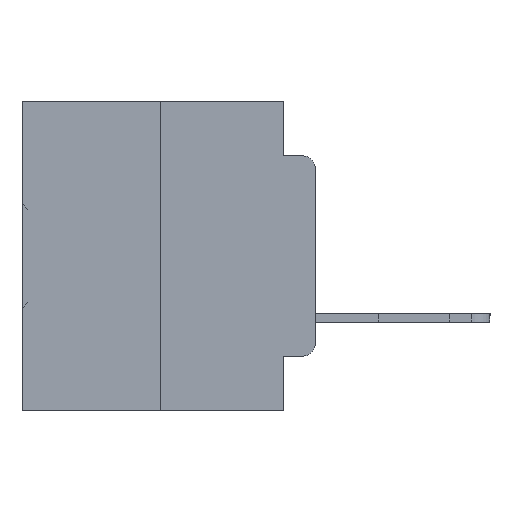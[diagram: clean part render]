
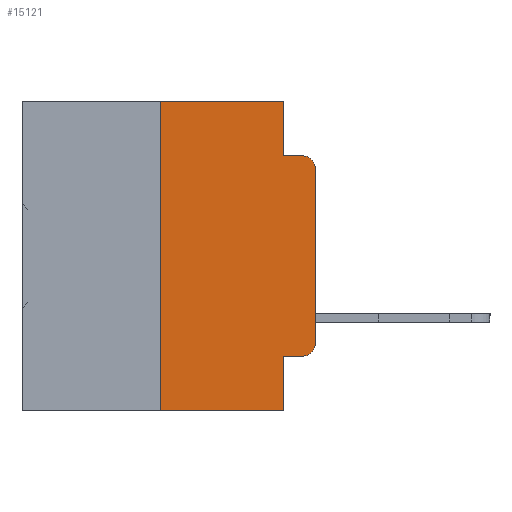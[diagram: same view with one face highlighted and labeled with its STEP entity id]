
A CAD part, left-side view. The second image highlights one B-rep face of the part: STEP entity #15121.
In plain terms, the highlighted planar face has unit normal (-1, 0, 0).
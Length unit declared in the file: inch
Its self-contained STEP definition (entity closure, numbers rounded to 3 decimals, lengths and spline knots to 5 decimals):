
#551 = DIRECTION ( 'NONE',  ( 0., 0., 1. ) ) ;
#1004 = VERTEX_POINT ( 'NONE', #1181 ) ;
#1014 = CARTESIAN_POINT ( 'NONE',  ( 0., 0.051, -0.5 ) ) ;
#1134 = ORIENTED_EDGE ( 'NONE', *, *, #14506, .F. ) ;
#1181 = CARTESIAN_POINT ( 'NONE',  ( 0., 0.051, 0. ) ) ;
#1571 = EDGE_CURVE ( 'NONE', #15474, #32613, #20621, .T. ) ;
#1595 = CARTESIAN_POINT ( 'NONE',  ( 0., 0.051, 0. ) ) ;
#1701 = LINE ( 'NONE', #3134, #15509 ) ;
#2560 = CARTESIAN_POINT ( 'NONE',  ( 0., 0., 0. ) ) ;
#3134 = CARTESIAN_POINT ( 'NONE',  ( 0., 0.051, 0. ) ) ;
#4135 = ORIENTED_EDGE ( 'NONE', *, *, #34524, .T. ) ;
#4772 = DIRECTION ( 'NONE',  ( -1., 0., 0. ) ) ;
#4811 = EDGE_CURVE ( 'NONE', #16087, #28136, #8216, .T. ) ;
#5241 = EDGE_CURVE ( 'NONE', #15474, #28136, #1701, .T. ) ;
#6023 = VECTOR ( 'NONE', #12230, 39.37008 ) ;
#6100 = VECTOR ( 'NONE', #30065, 39.37008 ) ;
#6798 = DIRECTION ( 'NONE',  ( 0., -1., 0. ) ) ;
#7503 = CARTESIAN_POINT ( 'NONE',  ( 0., 0.051, -0.4115 ) ) ;
#8216 = LINE ( 'NONE', #17847, #21901 ) ;
#10255 = PLANE ( 'NONE',  #13901 ) ;
#10824 = EDGE_CURVE ( 'NONE', #16087, #13221, #30227, .T. ) ;
#11546 = CARTESIAN_POINT ( 'NONE',  ( 0., 0.25, 0. ) ) ;
#11684 = CARTESIAN_POINT ( 'NONE',  ( 0., 0.02, -0.4115 ) ) ;
#12230 = DIRECTION ( 'NONE',  ( 0., -1., 0. ) ) ;
#12981 = DIRECTION ( 'NONE',  ( 1., 0., 0. ) ) ;
#13137 = VERTEX_POINT ( 'NONE', #23267 ) ;
#13175 = EDGE_LOOP ( 'NONE', ( #4135, #26009, #34906, #1134, #15831, #23039, #24764, #31953, #18384, #19236 ) ) ;
#13221 = VERTEX_POINT ( 'NONE', #18149 ) ;
#13512 = DIRECTION ( 'NONE',  ( 0., 0., 1. ) ) ;
#13901 = AXIS2_PLACEMENT_3D ( 'NONE', #15553, #12981, #32032 ) ;
#14374 = CARTESIAN_POINT ( 'NONE',  ( 0., 0., -0.3915 ) ) ;
#14460 = LINE ( 'NONE', #2560, #28094 ) ;
#14506 = EDGE_CURVE ( 'NONE', #1004, #29468, #30001, .T. ) ;
#15121 = ADVANCED_FACE ( 'NONE', ( #32911 ), #10255, .F. ) ;
#15203 = LINE ( 'NONE', #27362, #6100 ) ;
#15474 = VERTEX_POINT ( 'NONE', #7503 ) ;
#15509 = VECTOR ( 'NONE', #22340, 39.37008 ) ;
#15553 = CARTESIAN_POINT ( 'NONE',  ( 0., 0.473, 0. ) ) ;
#15802 = DIRECTION ( 'NONE',  ( 0., -1., 0. ) ) ;
#15831 = ORIENTED_EDGE ( 'NONE', *, *, #35040, .F. ) ;
#16087 = VERTEX_POINT ( 'NONE', #18883 ) ;
#16089 = DIRECTION ( 'NONE',  ( -1., 0., 0. ) ) ;
#17183 = VECTOR ( 'NONE', #15802, 39.37008 ) ;
#17699 = VERTEX_POINT ( 'NONE', #17917 ) ;
#17847 = CARTESIAN_POINT ( 'NONE',  ( 0., 0.473, -0.5 ) ) ;
#17917 = CARTESIAN_POINT ( 'NONE',  ( 0., 0., -0.1085 ) ) ;
#18020 = LINE ( 'NONE', #26697, #17183 ) ;
#18149 = CARTESIAN_POINT ( 'NONE',  ( 0., 0.25, 0. ) ) ;
#18384 = ORIENTED_EDGE ( 'NONE', *, *, #1571, .T. ) ;
#18444 = VERTEX_POINT ( 'NONE', #14374 ) ;
#18883 = CARTESIAN_POINT ( 'NONE',  ( 0., 0.25, -0.5 ) ) ;
#19236 = ORIENTED_EDGE ( 'NONE', *, *, #31574, .T. ) ;
#20198 = AXIS2_PLACEMENT_3D ( 'NONE', #32330, #16089, #35048 ) ;
#20621 = LINE ( 'NONE', #34000, #6023 ) ;
#21212 = CARTESIAN_POINT ( 'NONE',  ( 0., 0.02, -0.1085 ) ) ;
#21901 = VECTOR ( 'NONE', #6798, 39.37008 ) ;
#22340 = DIRECTION ( 'NONE',  ( 0., 0., -1. ) ) ;
#22773 = VECTOR ( 'NONE', #34306, 39.37008 ) ;
#23039 = ORIENTED_EDGE ( 'NONE', *, *, #10824, .F. ) ;
#23267 = CARTESIAN_POINT ( 'NONE',  ( 0., 0.02, -0.0885 ) ) ;
#23972 = DIRECTION ( 'NONE',  ( 0., 0., -1. ) ) ;
#24764 = ORIENTED_EDGE ( 'NONE', *, *, #4811, .T. ) ;
#25140 = CARTESIAN_POINT ( 'NONE',  ( 0., 0.051, -0.0885 ) ) ;
#25438 = EDGE_CURVE ( 'NONE', #29468, #13137, #15203, .T. ) ;
#25871 = AXIS2_PLACEMENT_3D ( 'NONE', #21212, #4772, #23972 ) ;
#26009 = ORIENTED_EDGE ( 'NONE', *, *, #30885, .T. ) ;
#26697 = CARTESIAN_POINT ( 'NONE',  ( 0., 0.473, 0. ) ) ;
#27362 = CARTESIAN_POINT ( 'NONE',  ( 0., 0.051, -0.0885 ) ) ;
#27489 = CIRCLE ( 'NONE', #25871, 0.02 ) ;
#28094 = VECTOR ( 'NONE', #13512, 39.37008 ) ;
#28136 = VERTEX_POINT ( 'NONE', #1014 ) ;
#29384 = VECTOR ( 'NONE', #551, 39.37008 ) ;
#29468 = VERTEX_POINT ( 'NONE', #25140 ) ;
#30001 = LINE ( 'NONE', #1595, #22773 ) ;
#30065 = DIRECTION ( 'NONE',  ( 0., -1., 0. ) ) ;
#30227 = LINE ( 'NONE', #11546, #29384 ) ;
#30885 = EDGE_CURVE ( 'NONE', #17699, #13137, #27489, .T. ) ;
#31574 = EDGE_CURVE ( 'NONE', #32613, #18444, #34183, .T. ) ;
#31953 = ORIENTED_EDGE ( 'NONE', *, *, #5241, .F. ) ;
#32032 = DIRECTION ( 'NONE',  ( 0., 0., -1. ) ) ;
#32330 = CARTESIAN_POINT ( 'NONE',  ( 0., 0.02, -0.3915 ) ) ;
#32613 = VERTEX_POINT ( 'NONE', #11684 ) ;
#32911 = FACE_OUTER_BOUND ( 'NONE', #13175, .T. ) ;
#34000 = CARTESIAN_POINT ( 'NONE',  ( 0., 0.051, -0.4115 ) ) ;
#34183 = CIRCLE ( 'NONE', #20198, 0.02 ) ;
#34306 = DIRECTION ( 'NONE',  ( 0., 0., -1. ) ) ;
#34524 = EDGE_CURVE ( 'NONE', #18444, #17699, #14460, .T. ) ;
#34906 = ORIENTED_EDGE ( 'NONE', *, *, #25438, .F. ) ;
#35040 = EDGE_CURVE ( 'NONE', #13221, #1004, #18020, .T. ) ;
#35048 = DIRECTION ( 'NONE',  ( 0., 0., -1. ) ) ;
